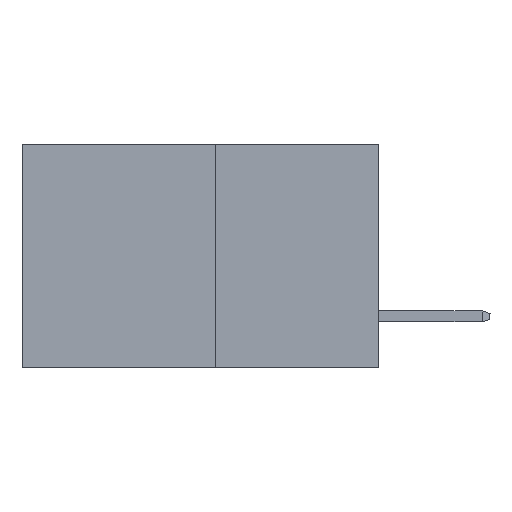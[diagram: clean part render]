
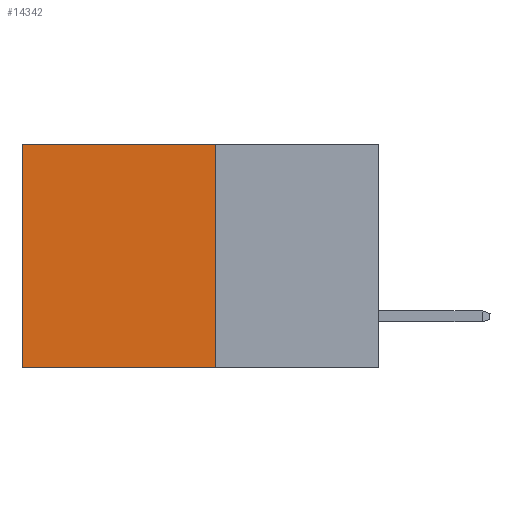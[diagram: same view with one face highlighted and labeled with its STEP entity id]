
A CAD part, left-side view. The second image highlights one B-rep face of the part: STEP entity #14342.
In plain terms, the highlighted planar face has unit normal (-1, 0, 0).
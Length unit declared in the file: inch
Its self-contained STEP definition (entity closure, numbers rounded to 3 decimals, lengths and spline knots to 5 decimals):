
#346 = LINE ( 'NONE', #10946, #12339 ) ;
#739 = EDGE_CURVE ( 'NONE', #8226, #7209, #11624, .T. ) ;
#772 = DIRECTION ( 'NONE',  ( 0., 0., -1. ) ) ;
#1202 = ORIENTED_EDGE ( 'NONE', *, *, #12415, .T. ) ;
#1887 = PLANE ( 'NONE',  #5702 ) ;
#3483 = DIRECTION ( 'NONE',  ( 0., 0., -1. ) ) ;
#4159 = CARTESIAN_POINT ( 'NONE',  ( 0.277, 0.27, -0.37 ) ) ;
#5247 = VERTEX_POINT ( 'NONE', #13454 ) ;
#5661 = ORIENTED_EDGE ( 'NONE', *, *, #739, .F. ) ;
#5702 = AXIS2_PLACEMENT_3D ( 'NONE', #4159, #7594, #772 ) ;
#6546 = CARTESIAN_POINT ( 'NONE',  ( 0.277, 0.59, -0.37 ) ) ;
#6835 = DIRECTION ( 'NONE',  ( 0., 1., 0. ) ) ;
#7209 = VERTEX_POINT ( 'NONE', #6546 ) ;
#7594 = DIRECTION ( 'NONE',  ( 1., 0., 0. ) ) ;
#7965 = VECTOR ( 'NONE', #3483, 39.37008 ) ;
#8226 = VERTEX_POINT ( 'NONE', #9468 ) ;
#8350 = EDGE_CURVE ( 'NONE', #5247, #8226, #346, .T. ) ;
#8701 = VECTOR ( 'NONE', #6835, 39.37008 ) ;
#9003 = ORIENTED_EDGE ( 'NONE', *, *, #8350, .F. ) ;
#9132 = CARTESIAN_POINT ( 'NONE',  ( 0.277, 0.59, -0.37 ) ) ;
#9250 = DIRECTION ( 'NONE',  ( 0., 1., 0. ) ) ;
#9468 = CARTESIAN_POINT ( 'NONE',  ( 0.277, 0.27, -0.37 ) ) ;
#9508 = VECTOR ( 'NONE', #9250, 39.37008 ) ;
#9533 = CARTESIAN_POINT ( 'NONE',  ( 0.277, 0.27, -0.37 ) ) ;
#10820 = EDGE_LOOP ( 'NONE', ( #14094, #5661, #9003, #1202 ) ) ;
#10935 = LINE ( 'NONE', #9132, #7965 ) ;
#10946 = CARTESIAN_POINT ( 'NONE',  ( 0.277, 0.27, -0.37 ) ) ;
#11296 = EDGE_CURVE ( 'NONE', #13697, #7209, #10935, .T. ) ;
#11624 = LINE ( 'NONE', #9533, #8701 ) ;
#12001 = DIRECTION ( 'NONE',  ( 0., 0., -1. ) ) ;
#12128 = FACE_OUTER_BOUND ( 'NONE', #10820, .T. ) ;
#12339 = VECTOR ( 'NONE', #12001, 39.37008 ) ;
#12370 = LINE ( 'NONE', #13551, #9508 ) ;
#12415 = EDGE_CURVE ( 'NONE', #5247, #13697, #12370, .T. ) ;
#13454 = CARTESIAN_POINT ( 'NONE',  ( 0.277, 0.27, 0. ) ) ;
#13551 = CARTESIAN_POINT ( 'NONE',  ( 0.277, 0.27, 0. ) ) ;
#13697 = VERTEX_POINT ( 'NONE', #13973 ) ;
#13973 = CARTESIAN_POINT ( 'NONE',  ( 0.277, 0.59, 0. ) ) ;
#14094 = ORIENTED_EDGE ( 'NONE', *, *, #11296, .T. ) ;
#14342 = ADVANCED_FACE ( 'NONE', ( #12128 ), #1887, .F. ) ;
